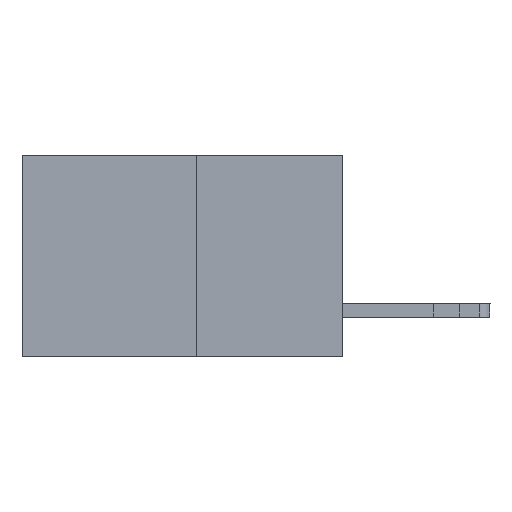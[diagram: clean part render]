
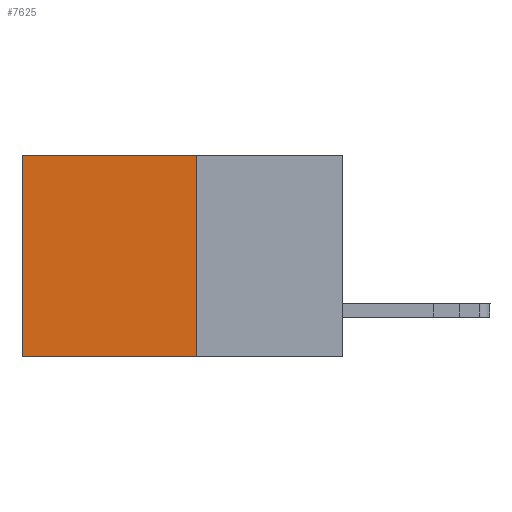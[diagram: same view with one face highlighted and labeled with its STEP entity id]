
A CAD part, left-side view. The second image highlights one B-rep face of the part: STEP entity #7625.
In plain terms, the highlighted planar face has unit normal (-1, 0, 0).
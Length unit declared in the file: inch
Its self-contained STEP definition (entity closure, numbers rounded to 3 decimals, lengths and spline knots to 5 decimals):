
#2661 = VERTEX_POINT ( 'NONE', #21378 ) ;
#3626 = ORIENTED_EDGE ( 'NONE', *, *, #23430, .T. ) ;
#3849 = ORIENTED_EDGE ( 'NONE', *, *, #20767, .F. ) ;
#4307 = EDGE_LOOP ( 'NONE', ( #5109, #3849, #5357, #3626 ) ) ;
#5109 = ORIENTED_EDGE ( 'NONE', *, *, #9525, .T. ) ;
#5357 = ORIENTED_EDGE ( 'NONE', *, *, #16933, .F. ) ;
#6544 = CARTESIAN_POINT ( 'NONE',  ( 0.277, 0.27, -0.37 ) ) ;
#7278 = VECTOR ( 'NONE', #16233, 39.37008 ) ;
#7625 = ADVANCED_FACE ( 'NONE', ( #11574 ), #18668, .F. ) ;
#7927 = CARTESIAN_POINT ( 'NONE',  ( 0.277, 0.59, -0.37 ) ) ;
#8199 = VERTEX_POINT ( 'NONE', #14481 ) ;
#8906 = LINE ( 'NONE', #9549, #13872 ) ;
#9038 = CARTESIAN_POINT ( 'NONE',  ( 0.277, 0.59, -0.37 ) ) ;
#9525 = EDGE_CURVE ( 'NONE', #8199, #19711, #18974, .T. ) ;
#9549 = CARTESIAN_POINT ( 'NONE',  ( 0.277, 0.27, -0.37 ) ) ;
#9729 = VECTOR ( 'NONE', #10861, 39.37008 ) ;
#10861 = DIRECTION ( 'NONE',  ( 0., 0., -1. ) ) ;
#11343 = DIRECTION ( 'NONE',  ( 0., 0., -1. ) ) ;
#11357 = DIRECTION ( 'NONE',  ( 0., 0., -1. ) ) ;
#11574 = FACE_OUTER_BOUND ( 'NONE', #4307, .T. ) ;
#13269 = DIRECTION ( 'NONE',  ( 0., 1., 0. ) ) ;
#13872 = VECTOR ( 'NONE', #13269, 39.37008 ) ;
#14481 = CARTESIAN_POINT ( 'NONE',  ( 0.277, 0.59, 0. ) ) ;
#16233 = DIRECTION ( 'NONE',  ( 0., 1., 0. ) ) ;
#16673 = VECTOR ( 'NONE', #11357, 39.37008 ) ;
#16811 = CARTESIAN_POINT ( 'NONE',  ( 0.277, 0.27, -0.37 ) ) ;
#16933 = EDGE_CURVE ( 'NONE', #2661, #22250, #17258, .T. ) ;
#17199 = LINE ( 'NONE', #20138, #7278 ) ;
#17258 = LINE ( 'NONE', #16811, #16673 ) ;
#18203 = AXIS2_PLACEMENT_3D ( 'NONE', #20570, #22433, #11343 ) ;
#18668 = PLANE ( 'NONE',  #18203 ) ;
#18974 = LINE ( 'NONE', #9038, #9729 ) ;
#19711 = VERTEX_POINT ( 'NONE', #7927 ) ;
#20138 = CARTESIAN_POINT ( 'NONE',  ( 0.277, 0.27, 0. ) ) ;
#20570 = CARTESIAN_POINT ( 'NONE',  ( 0.277, 0.27, -0.37 ) ) ;
#20767 = EDGE_CURVE ( 'NONE', #22250, #19711, #8906, .T. ) ;
#21378 = CARTESIAN_POINT ( 'NONE',  ( 0.277, 0.27, 0. ) ) ;
#22250 = VERTEX_POINT ( 'NONE', #6544 ) ;
#22433 = DIRECTION ( 'NONE',  ( 1., 0., 0. ) ) ;
#23430 = EDGE_CURVE ( 'NONE', #2661, #8199, #17199, .T. ) ;
